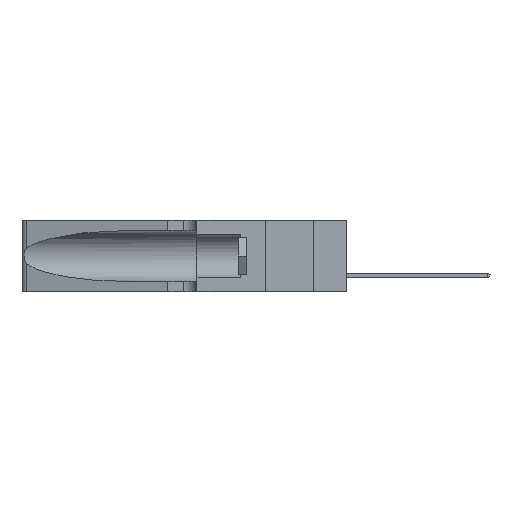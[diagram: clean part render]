
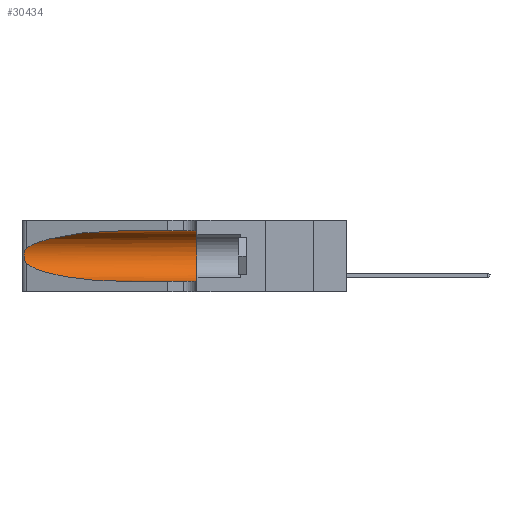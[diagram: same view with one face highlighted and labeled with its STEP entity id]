
A CAD part, left-side view. The second image highlights one B-rep face of the part: STEP entity #30434.
In plain terms, the highlighted cylindrical face has radius 3.308 mm (diameter 6.617 mm), a partial arc.
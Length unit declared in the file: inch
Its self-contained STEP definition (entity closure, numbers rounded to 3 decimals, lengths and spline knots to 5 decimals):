
#199 = CARTESIAN_POINT ( 'NONE',  ( 0.25487, 1.22718, 0.22369 ) ) ;
#2293 = CARTESIAN_POINT ( 'NONE',  ( 0.25639, 1.23184, 0.21858 ) ) ;
#2533 = CARTESIAN_POINT ( 'NONE',  ( 0.1305, 0.72297, 0.05475 ) ) ;
#2707 = CIRCLE ( 'NONE', #19362, 0.13025 ) ;
#2738 = VERTEX_POINT ( 'NONE', #15745 ) ;
#3006 = CARTESIAN_POINT ( 'NONE',  ( 0.1305, 1.61858, 0.31525 ) ) ;
#3415 = VERTEX_POINT ( 'NONE', #14309 ) ;
#3537 = AXIS2_PLACEMENT_3D ( 'NONE', #15520, #15742, #8212 ) ;
#4115 = ORIENTED_EDGE ( 'NONE', *, *, #9240, .T. ) ;
#4635 = VERTEX_POINT ( 'NONE', #199 ) ;
#4759 = CARTESIAN_POINT ( 'NONE',  ( 0.2373, 1.15595, 0.08982 ) ) ;
#4874 = CARTESIAN_POINT ( 'NONE',  ( 0.25487, 1.22718, 0.22369 ) ) ;
#6016 = CARTESIAN_POINT ( 'NONE',  ( 0.25487, 1.22718, 0.14631 ) ) ;
#6289 = CARTESIAN_POINT ( 'NONE',  ( 0.1305, 0.72297, 0.31525 ) ) ;
#6595 = CARTESIAN_POINT ( 'NONE',  ( 0.1305, 1.61858, 0.05475 ) ) ;
#6899 = VERTEX_POINT ( 'NONE', #10907 ) ;
#7817 = ORIENTED_EDGE ( 'NONE', *, *, #13174, .F. ) ;
#8212 = DIRECTION ( 'NONE',  ( 0., 0., -1. ) ) ;
#8686 = CARTESIAN_POINT ( 'NONE',  ( 0.2373, 1.15595, 0.28018 ) ) ;
#9240 = EDGE_CURVE ( 'NONE', #3415, #4635, #19164, .T. ) ;
#10040 = VERTEX_POINT ( 'NONE', #6016 ) ;
#10069 = CARTESIAN_POINT ( 'NONE',  ( 0.25787, 1.23484, 0.2124 ) ) ;
#10173 = CARTESIAN_POINT ( 'NONE',  ( 0.26075, 1.23896, 0.19203 ) ) ;
#10337 = CYLINDRICAL_SURFACE ( 'NONE', #3537, 0.13025 ) ;
#10907 = CARTESIAN_POINT ( 'NONE',  ( 0.1305, 0.35, 0.31525 ) ) ;
#12615 = CARTESIAN_POINT ( 'NONE',  ( 0.25856, 1.23593, 0.16098 ) ) ;
#12840 = CARTESIAN_POINT ( 'NONE',  ( 0.25639, 1.23186, 0.15144 ) ) ;
#13174 = EDGE_CURVE ( 'NONE', #6899, #2738, #2707, .T. ) ;
#13312 = EDGE_CURVE ( 'NONE', #4635, #10040, #23795, .T. ) ;
#13347 = EDGE_CURVE ( 'NONE', #10040, #29627, #31861, .T. ) ;
#14058 = CARTESIAN_POINT ( 'NONE',  ( 0.18966, 0.96281, 0.31525 ) ) ;
#14309 = CARTESIAN_POINT ( 'NONE',  ( 0.1305, 0.72297, 0.31525 ) ) ;
#14788 = ORIENTED_EDGE ( 'NONE', *, *, #13347, .T. ) ;
#15413 = EDGE_CURVE ( 'NONE', #3415, #6899, #24541, .T. ) ;
#15488 = CARTESIAN_POINT ( 'NONE',  ( 0.25487, 1.22718, 0.14631 ) ) ;
#15520 = CARTESIAN_POINT ( 'NONE',  ( 0.1305, 1.61858, 0.185 ) ) ;
#15742 = DIRECTION ( 'NONE',  ( 0., -1., 0. ) ) ;
#15745 = CARTESIAN_POINT ( 'NONE',  ( 0.1305, 0.35, 0.05475 ) ) ;
#16869 = LINE ( 'NONE', #6595, #17695 ) ;
#17455 = VECTOR ( 'NONE', #31969, 39.37008 ) ;
#17586 = CARTESIAN_POINT ( 'NONE',  ( 0.1305, 0.35, 0.185 ) ) ;
#17695 = VECTOR ( 'NONE', #22249, 39.37008 ) ;
#17809 = DIRECTION ( 'NONE',  ( 0., 1., 0. ) ) ;
#18181 = FACE_OUTER_BOUND ( 'NONE', #31898, .T. ) ;
#18351 = CARTESIAN_POINT ( 'NONE',  ( 0.25854, 1.2359, 0.20912 ) ) ;
#19164 =( BOUNDED_CURVE ( )  B_SPLINE_CURVE ( 3, ( #6289, #14058, #8686, #27537 ),
 .UNSPECIFIED., .F., .F. ) 
 B_SPLINE_CURVE_WITH_KNOTS ( ( 4, 4 ),
 ( 1.5708, 2.84003 ),
 .UNSPECIFIED. ) 
 CURVE ( )  GEOMETRIC_REPRESENTATION_ITEM ( )  RATIONAL_B_SPLINE_CURVE ( ( 1., 0.87, 0.87, 1. ) ) 
 REPRESENTATION_ITEM ( '' )  );
#19362 = AXIS2_PLACEMENT_3D ( 'NONE', #17586, #17809, #28452 ) ;
#20625 = CARTESIAN_POINT ( 'NONE',  ( 0.26017, 1.23833, 0.17102 ) ) ;
#20840 = CARTESIAN_POINT ( 'NONE',  ( 0.26018, 1.23835, 0.19895 ) ) ;
#21759 = CARTESIAN_POINT ( 'NONE',  ( 0.1305, 0.72297, 0.05475 ) ) ;
#22249 = DIRECTION ( 'NONE',  ( 0., -1., 0. ) ) ;
#23414 = CARTESIAN_POINT ( 'NONE',  ( 0.25555, 1.22994, 0.2215 ) ) ;
#23795 = B_SPLINE_CURVE_WITH_KNOTS ( 'NONE', 3,
 ( #4874, #23414, #2293, #10069, #18351, #20840, #10173, #28567, #20625, #12615, #26107, #12840, #31387, #15488 ),
 .UNSPECIFIED., .F., .F.,
 ( 4, 2, 2, 2, 2, 2, 4 ),
 ( 0., 0.00027, 0.00053, 0.00107, 0.0016, 0.00187, 0.00214 ),
 .UNSPECIFIED. ) ;
#24541 = LINE ( 'NONE', #3006, #17455 ) ;
#26107 = CARTESIAN_POINT ( 'NONE',  ( 0.25789, 1.23486, 0.15765 ) ) ;
#26517 = ORIENTED_EDGE ( 'NONE', *, *, #32868, .T. ) ;
#26606 = ORIENTED_EDGE ( 'NONE', *, *, #15413, .F. ) ;
#26937 = ORIENTED_EDGE ( 'NONE', *, *, #13312, .T. ) ;
#27537 = CARTESIAN_POINT ( 'NONE',  ( 0.25487, 1.22718, 0.22369 ) ) ;
#28452 = DIRECTION ( 'NONE',  ( 0., 0., 1. ) ) ;
#28567 = CARTESIAN_POINT ( 'NONE',  ( 0.26075, 1.23896, 0.178 ) ) ;
#29627 = VERTEX_POINT ( 'NONE', #21759 ) ;
#30434 = ADVANCED_FACE ( 'NONE', ( #18181 ), #10337, .F. ) ;
#31172 = CARTESIAN_POINT ( 'NONE',  ( 0.25487, 1.22718, 0.14631 ) ) ;
#31387 = CARTESIAN_POINT ( 'NONE',  ( 0.25555, 1.22993, 0.14849 ) ) ;
#31861 =( BOUNDED_CURVE ( )  B_SPLINE_CURVE ( 3, ( #31172, #4759, #34265, #2533 ),
 .UNSPECIFIED., .F., .F. ) 
 B_SPLINE_CURVE_WITH_KNOTS ( ( 4, 4 ),
 ( 3.44316, 4.71239 ),
 .UNSPECIFIED. ) 
 CURVE ( )  GEOMETRIC_REPRESENTATION_ITEM ( )  RATIONAL_B_SPLINE_CURVE ( ( 1., 0.87, 0.87, 1. ) ) 
 REPRESENTATION_ITEM ( '' )  );
#31898 = EDGE_LOOP ( 'NONE', ( #4115, #26937, #14788, #26517, #7817, #26606 ) ) ;
#31969 = DIRECTION ( 'NONE',  ( 0., -1., 0. ) ) ;
#32868 = EDGE_CURVE ( 'NONE', #29627, #2738, #16869, .T. ) ;
#34265 = CARTESIAN_POINT ( 'NONE',  ( 0.18966, 0.96281, 0.05475 ) ) ;
